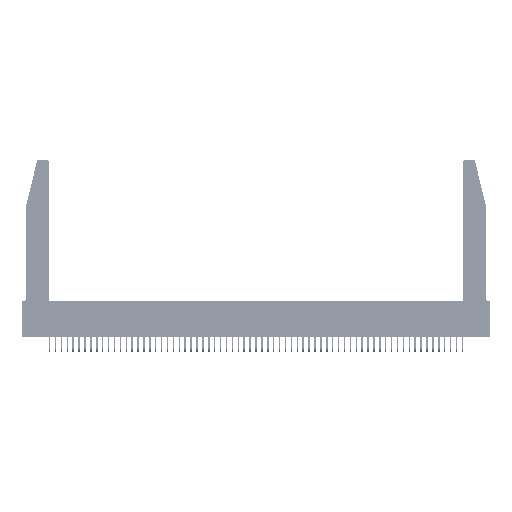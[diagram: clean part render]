
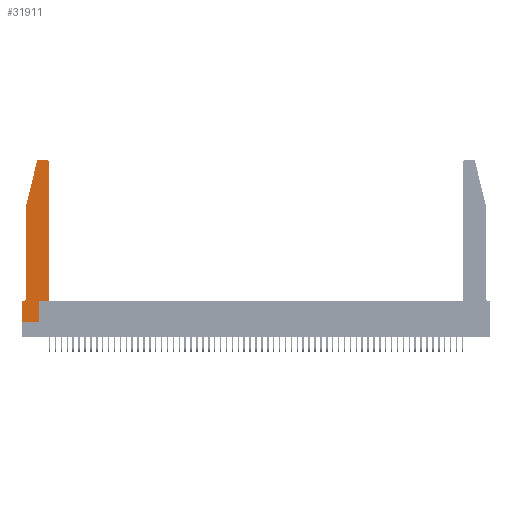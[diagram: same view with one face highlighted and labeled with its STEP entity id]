
A CAD part, top view. The second image highlights one B-rep face of the part: STEP entity #31911.
In plain terms, the highlighted planar face has unit normal (0, 0, 1).
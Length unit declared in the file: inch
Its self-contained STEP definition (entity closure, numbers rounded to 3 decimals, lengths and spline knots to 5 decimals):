
#757 = VECTOR ( 'NONE', #40182, 39.37008 ) ;
#968 = EDGE_CURVE ( 'NONE', #42775, #7937, #11906, .T. ) ;
#1397 = LINE ( 'NONE', #48887, #13359 ) ;
#1767 = CARTESIAN_POINT ( 'NONE',  ( 0.4205, 2.75, 0.37 ) ) ;
#1824 = CARTESIAN_POINT ( 'NONE',  ( 0., 0.35, 0.37 ) ) ;
#2090 = VECTOR ( 'NONE', #48992, 39.37008 ) ;
#2255 = DIRECTION ( 'NONE',  ( 1., 0., 0. ) ) ;
#2282 = CARTESIAN_POINT ( 'NONE',  ( 0.284, 2.75, 0.37 ) ) ;
#2991 = ORIENTED_EDGE ( 'NONE', *, *, #23353, .T. ) ;
#3179 = CARTESIAN_POINT ( 'NONE',  ( 0.0055, 0.35, 0.37 ) ) ;
#4124 = CARTESIAN_POINT ( 'NONE',  ( 0.4505, 0.35, 0.37 ) ) ;
#4927 = DIRECTION ( 'NONE',  ( 1., 0., 0. ) ) ;
#5376 = LINE ( 'NONE', #50296, #15901 ) ;
#5803 = CIRCLE ( 'NONE', #7929, 0.03 ) ;
#6361 = DIRECTION ( 'NONE',  ( 0., 0., 1. ) ) ;
#7464 = CARTESIAN_POINT ( 'NONE',  ( 0.2865, 0., 0.37 ) ) ;
#7929 = AXIS2_PLACEMENT_3D ( 'NONE', #56112, #29302, #2255 ) ;
#7937 = VERTEX_POINT ( 'NONE', #41803 ) ;
#8131 = ORIENTED_EDGE ( 'NONE', *, *, #37022, .T. ) ;
#8474 = AXIS2_PLACEMENT_3D ( 'NONE', #15008, #46555, #19575 ) ;
#8575 = CARTESIAN_POINT ( 'NONE',  ( 0.2605, 2.75, 0.37 ) ) ;
#9446 = CARTESIAN_POINT ( 'NONE',  ( 0., 0., 0.37 ) ) ;
#9831 = EDGE_CURVE ( 'NONE', #23551, #14670, #11313, .T. ) ;
#10089 = ORIENTED_EDGE ( 'NONE', *, *, #20642, .T. ) ;
#10492 = EDGE_CURVE ( 'NONE', #7937, #20504, #1397, .T. ) ;
#10793 = CIRCLE ( 'NONE', #8474, 0.03 ) ;
#11313 = LINE ( 'NONE', #8575, #757 ) ;
#11906 = LINE ( 'NONE', #47768, #30888 ) ;
#12565 = LINE ( 'NONE', #49997, #23202 ) ;
#13359 = VECTOR ( 'NONE', #53376, 39.37008 ) ;
#14670 = VERTEX_POINT ( 'NONE', #2282 ) ;
#15008 = CARTESIAN_POINT ( 'NONE',  ( 0.4205, 2.72, 0.37 ) ) ;
#15069 = CARTESIAN_POINT ( 'NONE',  ( 0.4505, 2.72, 0.37 ) ) ;
#15901 = VECTOR ( 'NONE', #32452, 39.37008 ) ;
#16137 = ORIENTED_EDGE ( 'NONE', *, *, #40402, .T. ) ;
#16226 = DIRECTION ( 'NONE',  ( 0., 1., 0. ) ) ;
#17484 = CARTESIAN_POINT ( 'NONE',  ( 0.0755, 2., 0.37 ) ) ;
#17667 = VECTOR ( 'NONE', #19016, 39.37008 ) ;
#17933 = EDGE_LOOP ( 'NONE', ( #27384, #40284, #10089, #23826, #2991, #53986, #8131, #16137, #57888, #49662, #52056, #55014 ) ) ;
#18693 = DIRECTION ( 'NONE',  ( -0.239, -0.971, 0. ) ) ;
#19016 = DIRECTION ( 'NONE',  ( -1., 0., 0. ) ) ;
#19421 = EDGE_CURVE ( 'NONE', #40154, #40573, #29692, .T. ) ;
#19464 = VECTOR ( 'NONE', #4927, 39.37008 ) ;
#19575 = DIRECTION ( 'NONE',  ( 1., 0., 0. ) ) ;
#20504 = VERTEX_POINT ( 'NONE', #4124 ) ;
#20642 = EDGE_CURVE ( 'NONE', #21873, #21895, #12565, .T. ) ;
#21848 = CARTESIAN_POINT ( 'NONE',  ( 0.0755, 2., 0.37 ) ) ;
#21873 = VERTEX_POINT ( 'NONE', #57535 ) ;
#21895 = VERTEX_POINT ( 'NONE', #21848 ) ;
#22321 = CARTESIAN_POINT ( 'NONE',  ( 0.0055, 0.42, 0.37 ) ) ;
#23202 = VECTOR ( 'NONE', #18693, 39.37008 ) ;
#23353 = EDGE_CURVE ( 'NONE', #53655, #40154, #27125, .T. ) ;
#23551 = VERTEX_POINT ( 'NONE', #1767 ) ;
#23826 = ORIENTED_EDGE ( 'NONE', *, *, #33853, .T. ) ;
#26658 = AXIS2_PLACEMENT_3D ( 'NONE', #1824, #6361, #37958 ) ;
#26807 = LINE ( 'NONE', #32807, #37404 ) ;
#26859 = DIRECTION ( 'NONE',  ( -1., 0., 0. ) ) ;
#27125 = CIRCLE ( 'NONE', #31660, 0.07 ) ;
#27384 = ORIENTED_EDGE ( 'NONE', *, *, #9831, .T. ) ;
#27510 = VERTEX_POINT ( 'NONE', #36479 ) ;
#27775 = EDGE_CURVE ( 'NONE', #14670, #21873, #5803, .T. ) ;
#28865 = PLANE ( 'NONE',  #26658 ) ;
#29302 = DIRECTION ( 'NONE',  ( 0., 0., 1. ) ) ;
#29692 = LINE ( 'NONE', #50522, #17667 ) ;
#30888 = VECTOR ( 'NONE', #16226, 39.37008 ) ;
#31157 = VERTEX_POINT ( 'NONE', #15069 ) ;
#31660 = AXIS2_PLACEMENT_3D ( 'NONE', #22321, #53727, #26859 ) ;
#31862 = EDGE_CURVE ( 'NONE', #31157, #23551, #10793, .T. ) ;
#31911 = ADVANCED_FACE ( 'NONE', ( #43988 ), #28865, .T. ) ;
#32452 = DIRECTION ( 'NONE',  ( 0., -1., 0. ) ) ;
#32807 = CARTESIAN_POINT ( 'NONE',  ( 0.4505, 0.35, 0.37 ) ) ;
#33853 = EDGE_CURVE ( 'NONE', #21895, #53655, #48621, .T. ) ;
#36479 = CARTESIAN_POINT ( 'NONE',  ( 0., 0., 0.37 ) ) ;
#37022 = EDGE_CURVE ( 'NONE', #40573, #27510, #5376, .T. ) ;
#37404 = VECTOR ( 'NONE', #55080, 39.37008 ) ;
#37958 = DIRECTION ( 'NONE',  ( 1., 0., 0. ) ) ;
#40154 = VERTEX_POINT ( 'NONE', #3179 ) ;
#40182 = DIRECTION ( 'NONE',  ( -1., 0., 0. ) ) ;
#40284 = ORIENTED_EDGE ( 'NONE', *, *, #27775, .T. ) ;
#40402 = EDGE_CURVE ( 'NONE', #27510, #42775, #55294, .T. ) ;
#40573 = VERTEX_POINT ( 'NONE', #55402 ) ;
#41803 = CARTESIAN_POINT ( 'NONE',  ( 0.2865, 0.35, 0.37 ) ) ;
#42775 = VERTEX_POINT ( 'NONE', #7464 ) ;
#43988 = FACE_OUTER_BOUND ( 'NONE', #17933, .T. ) ;
#45583 = EDGE_CURVE ( 'NONE', #20504, #31157, #26807, .T. ) ;
#46555 = DIRECTION ( 'NONE',  ( 0., 0., 1. ) ) ;
#47768 = CARTESIAN_POINT ( 'NONE',  ( 0.2865, 0.35, 0.37 ) ) ;
#48621 = LINE ( 'NONE', #17484, #2090 ) ;
#48887 = CARTESIAN_POINT ( 'NONE',  ( 0.4505, 0.35, 0.37 ) ) ;
#48992 = DIRECTION ( 'NONE',  ( 0., -1., 0. ) ) ;
#49662 = ORIENTED_EDGE ( 'NONE', *, *, #10492, .T. ) ;
#49997 = CARTESIAN_POINT ( 'NONE',  ( 0.0755, 2., 0.37 ) ) ;
#50296 = CARTESIAN_POINT ( 'NONE',  ( 0., 0., 0.37 ) ) ;
#50522 = CARTESIAN_POINT ( 'NONE',  ( 0.0755, 0.35, 0.37 ) ) ;
#52056 = ORIENTED_EDGE ( 'NONE', *, *, #45583, .T. ) ;
#53376 = DIRECTION ( 'NONE',  ( 1., 0., 0. ) ) ;
#53655 = VERTEX_POINT ( 'NONE', #56506 ) ;
#53727 = DIRECTION ( 'NONE',  ( 0., 0., -1. ) ) ;
#53986 = ORIENTED_EDGE ( 'NONE', *, *, #19421, .T. ) ;
#55014 = ORIENTED_EDGE ( 'NONE', *, *, #31862, .T. ) ;
#55080 = DIRECTION ( 'NONE',  ( 0., 1., 0. ) ) ;
#55294 = LINE ( 'NONE', #9446, #19464 ) ;
#55402 = CARTESIAN_POINT ( 'NONE',  ( 0., 0.35, 0.37 ) ) ;
#56112 = CARTESIAN_POINT ( 'NONE',  ( 0.284, 2.72, 0.37 ) ) ;
#56506 = CARTESIAN_POINT ( 'NONE',  ( 0.0755, 0.42, 0.37 ) ) ;
#57535 = CARTESIAN_POINT ( 'NONE',  ( 0.25487, 2.72718, 0.37 ) ) ;
#57888 = ORIENTED_EDGE ( 'NONE', *, *, #968, .T. ) ;
